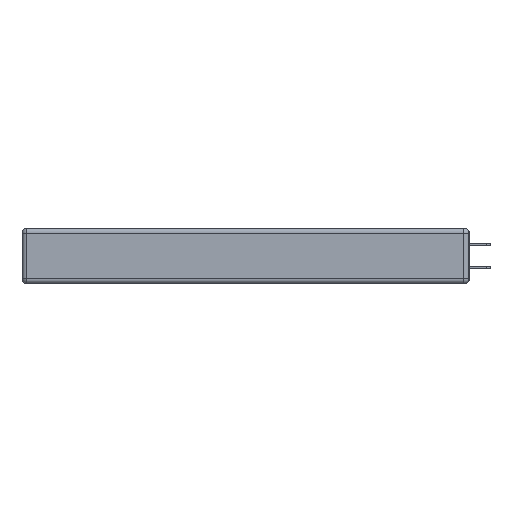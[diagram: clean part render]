
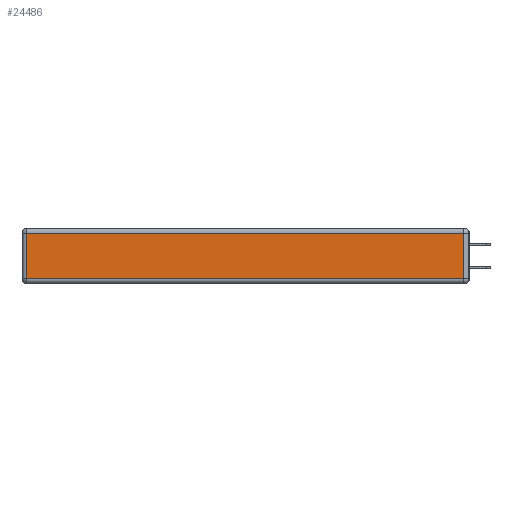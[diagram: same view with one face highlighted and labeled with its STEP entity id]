
A CAD part, left-side view. The second image highlights one B-rep face of the part: STEP entity #24486.
In plain terms, the highlighted planar face has unit normal (-1, 0, 0).
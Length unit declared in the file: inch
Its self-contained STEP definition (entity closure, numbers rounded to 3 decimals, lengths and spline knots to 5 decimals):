
#231 = LINE ( 'NONE', #15644, #31438 ) ;
#726 = DIRECTION ( 'NONE',  ( 0., -1., 0. ) ) ;
#2132 = ORIENTED_EDGE ( 'NONE', *, *, #3843, .T. ) ;
#2926 = VECTOR ( 'NONE', #25344, 39.37008 ) ;
#3843 = EDGE_CURVE ( 'NONE', #17241, #15214, #8451, .T. ) ;
#4642 = DIRECTION ( 'NONE',  ( 0., 0., 1. ) ) ;
#5922 = VECTOR ( 'NONE', #23939, 39.37008 ) ;
#6248 = CARTESIAN_POINT ( 'NONE',  ( 0., 0.03, -0.343 ) ) ;
#7192 = CARTESIAN_POINT ( 'NONE',  ( 0., 0.03, -0.03 ) ) ;
#7557 = CARTESIAN_POINT ( 'NONE',  ( 0., 2.75, -0.03 ) ) ;
#8451 = LINE ( 'NONE', #11652, #2926 ) ;
#9279 = EDGE_LOOP ( 'NONE', ( #22880, #13652, #27255, #2132 ) ) ;
#9695 = VERTEX_POINT ( 'NONE', #18247 ) ;
#9849 = DIRECTION ( 'NONE',  ( -1., 0., 0. ) ) ;
#9905 = LINE ( 'NONE', #6248, #5922 ) ;
#9949 = AXIS2_PLACEMENT_3D ( 'NONE', #29675, #9849, #4642 ) ;
#11652 = CARTESIAN_POINT ( 'NONE',  ( 0., 2.72, -0.343 ) ) ;
#12585 = EDGE_CURVE ( 'NONE', #9695, #13005, #9905, .T. ) ;
#13005 = VERTEX_POINT ( 'NONE', #7192 ) ;
#13652 = ORIENTED_EDGE ( 'NONE', *, *, #12585, .T. ) ;
#15202 = EDGE_CURVE ( 'NONE', #15214, #9695, #231, .T. ) ;
#15214 = VERTEX_POINT ( 'NONE', #23295 ) ;
#15644 = CARTESIAN_POINT ( 'NONE',  ( 0., 0., -0.313 ) ) ;
#16804 = LINE ( 'NONE', #7557, #19544 ) ;
#17241 = VERTEX_POINT ( 'NONE', #30716 ) ;
#18247 = CARTESIAN_POINT ( 'NONE',  ( 0., 0.03, -0.313 ) ) ;
#18615 = FACE_OUTER_BOUND ( 'NONE', #9279, .T. ) ;
#19544 = VECTOR ( 'NONE', #22247, 39.37008 ) ;
#22247 = DIRECTION ( 'NONE',  ( 0., 1., 0. ) ) ;
#22636 = PLANE ( 'NONE',  #9949 ) ;
#22880 = ORIENTED_EDGE ( 'NONE', *, *, #15202, .T. ) ;
#23295 = CARTESIAN_POINT ( 'NONE',  ( 0., 2.72, -0.313 ) ) ;
#23939 = DIRECTION ( 'NONE',  ( 0., 0., 1. ) ) ;
#24486 = ADVANCED_FACE ( 'NONE', ( #18615 ), #22636, .T. ) ;
#25344 = DIRECTION ( 'NONE',  ( 0., 0., -1. ) ) ;
#27255 = ORIENTED_EDGE ( 'NONE', *, *, #32115, .T. ) ;
#29675 = CARTESIAN_POINT ( 'NONE',  ( 0., 0., -0.343 ) ) ;
#30716 = CARTESIAN_POINT ( 'NONE',  ( 0., 2.72, -0.03 ) ) ;
#31438 = VECTOR ( 'NONE', #726, 39.37008 ) ;
#32115 = EDGE_CURVE ( 'NONE', #13005, #17241, #16804, .T. ) ;
